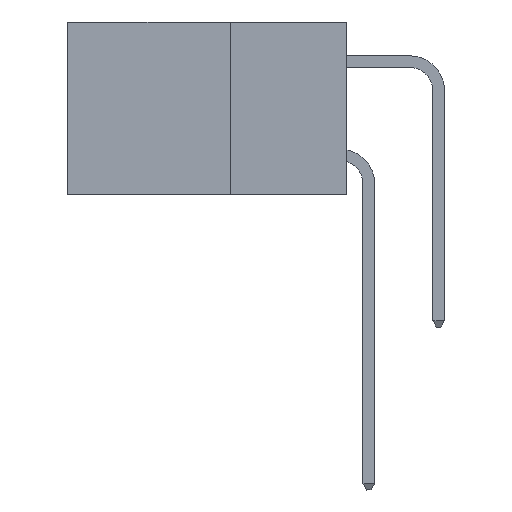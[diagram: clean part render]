
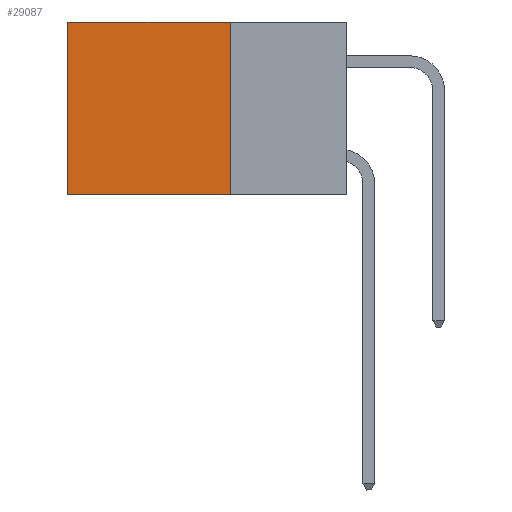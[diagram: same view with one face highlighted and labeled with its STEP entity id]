
A CAD part, left-side view. The second image highlights one B-rep face of the part: STEP entity #29087.
In plain terms, the highlighted planar face has unit normal (-1, 0, 0).
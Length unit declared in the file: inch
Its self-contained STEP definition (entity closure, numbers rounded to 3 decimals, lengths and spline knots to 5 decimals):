
#429 = DIRECTION ( 'NONE',  ( 1., 0., 0. ) ) ;
#1018 = ORIENTED_EDGE ( 'NONE', *, *, #24740, .F. ) ;
#1138 = VERTEX_POINT ( 'NONE', #27153 ) ;
#1941 = CARTESIAN_POINT ( 'NONE',  ( 0.2875, 0.25, 0. ) ) ;
#2842 = ORIENTED_EDGE ( 'NONE', *, *, #24292, .T. ) ;
#2929 = DIRECTION ( 'NONE',  ( 0., 0., -1. ) ) ;
#5381 = CARTESIAN_POINT ( 'NONE',  ( 0.2875, 0.25, 0. ) ) ;
#7909 = ORIENTED_EDGE ( 'NONE', *, *, #14766, .T. ) ;
#8093 = PLANE ( 'NONE',  #23974 ) ;
#8323 = LINE ( 'NONE', #16996, #13337 ) ;
#9321 = DIRECTION ( 'NONE',  ( 0., 0., -1. ) ) ;
#10023 = DIRECTION ( 'NONE',  ( 0., 0., -1. ) ) ;
#11693 = LINE ( 'NONE', #31334, #21791 ) ;
#13337 = VECTOR ( 'NONE', #30699, 39.37008 ) ;
#14766 = EDGE_CURVE ( 'NONE', #1138, #33463, #25927, .T. ) ;
#14800 = CARTESIAN_POINT ( 'NONE',  ( 0.2875, 0.6, 0. ) ) ;
#16996 = CARTESIAN_POINT ( 'NONE',  ( 0.2875, 0.25, -0.37 ) ) ;
#17714 = CARTESIAN_POINT ( 'NONE',  ( 0.2875, 0.6, -0.37 ) ) ;
#19525 = EDGE_LOOP ( 'NONE', ( #7909, #1018, #20604, #2842 ) ) ;
#20297 = VERTEX_POINT ( 'NONE', #23637 ) ;
#20604 = ORIENTED_EDGE ( 'NONE', *, *, #28116, .F. ) ;
#21153 = LINE ( 'NONE', #1941, #29868 ) ;
#21422 = CARTESIAN_POINT ( 'NONE',  ( 0.2875, 0.25, -0.37 ) ) ;
#21477 = FACE_OUTER_BOUND ( 'NONE', #19525, .T. ) ;
#21791 = VECTOR ( 'NONE', #23052, 39.37008 ) ;
#23052 = DIRECTION ( 'NONE',  ( 0., 1., 0. ) ) ;
#23637 = CARTESIAN_POINT ( 'NONE',  ( 0.2875, 0.25, 0. ) ) ;
#23974 = AXIS2_PLACEMENT_3D ( 'NONE', #5381, #429, #2929 ) ;
#24292 = EDGE_CURVE ( 'NONE', #20297, #1138, #11693, .T. ) ;
#24740 = EDGE_CURVE ( 'NONE', #27615, #33463, #8323, .T. ) ;
#25927 = LINE ( 'NONE', #14800, #32165 ) ;
#27153 = CARTESIAN_POINT ( 'NONE',  ( 0.2875, 0.6, 0. ) ) ;
#27615 = VERTEX_POINT ( 'NONE', #21422 ) ;
#28116 = EDGE_CURVE ( 'NONE', #20297, #27615, #21153, .T. ) ;
#29087 = ADVANCED_FACE ( 'NONE', ( #21477 ), #8093, .F. ) ;
#29868 = VECTOR ( 'NONE', #10023, 39.37008 ) ;
#30699 = DIRECTION ( 'NONE',  ( 0., 1., 0. ) ) ;
#31334 = CARTESIAN_POINT ( 'NONE',  ( 0.2875, 0.25, 0. ) ) ;
#32165 = VECTOR ( 'NONE', #9321, 39.37008 ) ;
#33463 = VERTEX_POINT ( 'NONE', #17714 ) ;
